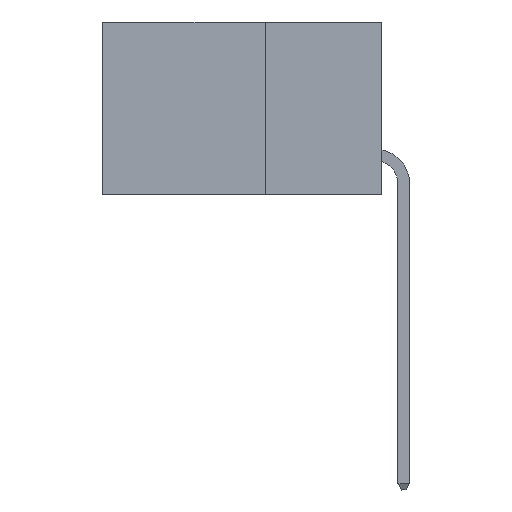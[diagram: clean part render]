
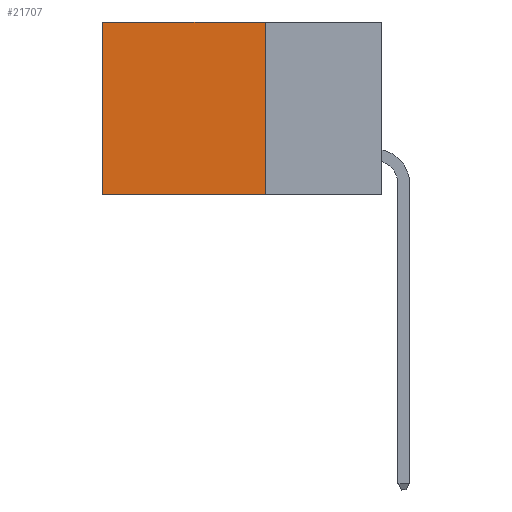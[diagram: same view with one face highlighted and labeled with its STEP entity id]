
A CAD part, left-side view. The second image highlights one B-rep face of the part: STEP entity #21707.
In plain terms, the highlighted planar face has unit normal (-1, 0, 0).
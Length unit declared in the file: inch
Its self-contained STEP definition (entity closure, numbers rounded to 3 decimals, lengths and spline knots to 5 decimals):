
#626 = VERTEX_POINT ( 'NONE', #19853 ) ;
#4046 = LINE ( 'NONE', #6961, #43062 ) ;
#4085 = DIRECTION ( 'NONE',  ( 0., 1., 0. ) ) ;
#4718 = AXIS2_PLACEMENT_3D ( 'NONE', #34856, #27438, #5078 ) ;
#4723 = LINE ( 'NONE', #39755, #32649 ) ;
#5078 = DIRECTION ( 'NONE',  ( 0., 0., -1. ) ) ;
#6961 = CARTESIAN_POINT ( 'NONE',  ( 0.2875, 0.25, -0.37 ) ) ;
#7255 = VERTEX_POINT ( 'NONE', #48941 ) ;
#9229 = VECTOR ( 'NONE', #10840, 39.37008 ) ;
#10840 = DIRECTION ( 'NONE',  ( 0., 0., -1. ) ) ;
#10898 = EDGE_CURVE ( 'NONE', #30153, #43231, #39766, .T. ) ;
#14242 = EDGE_CURVE ( 'NONE', #626, #7255, #22347, .T. ) ;
#16086 = EDGE_CURVE ( 'NONE', #43231, #7255, #4046, .T. ) ;
#16172 = PLANE ( 'NONE',  #4718 ) ;
#19853 = CARTESIAN_POINT ( 'NONE',  ( 0.2875, 0.6, 0. ) ) ;
#21707 = ADVANCED_FACE ( 'NONE', ( #34490 ), #16172, .F. ) ;
#22347 = LINE ( 'NONE', #41588, #9229 ) ;
#22600 = CARTESIAN_POINT ( 'NONE',  ( 0.2875, 0.25, 0. ) ) ;
#26489 = EDGE_LOOP ( 'NONE', ( #36538, #28931, #38723, #41474 ) ) ;
#26927 = EDGE_CURVE ( 'NONE', #30153, #626, #4723, .T. ) ;
#27438 = DIRECTION ( 'NONE',  ( 1., 0., 0. ) ) ;
#28931 = ORIENTED_EDGE ( 'NONE', *, *, #16086, .F. ) ;
#30153 = VERTEX_POINT ( 'NONE', #22600 ) ;
#30432 = CARTESIAN_POINT ( 'NONE',  ( 0.2875, 0.25, 0. ) ) ;
#32649 = VECTOR ( 'NONE', #36456, 39.37008 ) ;
#34490 = FACE_OUTER_BOUND ( 'NONE', #26489, .T. ) ;
#34856 = CARTESIAN_POINT ( 'NONE',  ( 0.2875, 0.25, 0. ) ) ;
#36456 = DIRECTION ( 'NONE',  ( 0., 1., 0. ) ) ;
#36538 = ORIENTED_EDGE ( 'NONE', *, *, #14242, .T. ) ;
#37314 = CARTESIAN_POINT ( 'NONE',  ( 0.2875, 0.25, -0.37 ) ) ;
#38723 = ORIENTED_EDGE ( 'NONE', *, *, #10898, .F. ) ;
#39755 = CARTESIAN_POINT ( 'NONE',  ( 0.2875, 0.25, 0. ) ) ;
#39766 = LINE ( 'NONE', #30432, #43901 ) ;
#41474 = ORIENTED_EDGE ( 'NONE', *, *, #26927, .T. ) ;
#41588 = CARTESIAN_POINT ( 'NONE',  ( 0.2875, 0.6, 0. ) ) ;
#41653 = DIRECTION ( 'NONE',  ( 0., 0., -1. ) ) ;
#43062 = VECTOR ( 'NONE', #4085, 39.37008 ) ;
#43231 = VERTEX_POINT ( 'NONE', #37314 ) ;
#43901 = VECTOR ( 'NONE', #41653, 39.37008 ) ;
#48941 = CARTESIAN_POINT ( 'NONE',  ( 0.2875, 0.6, -0.37 ) ) ;
